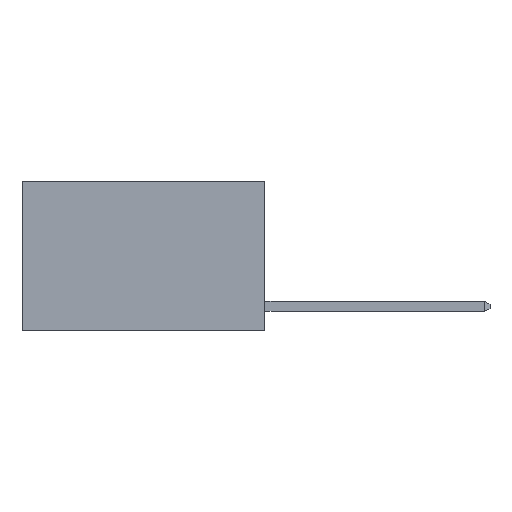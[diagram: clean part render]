
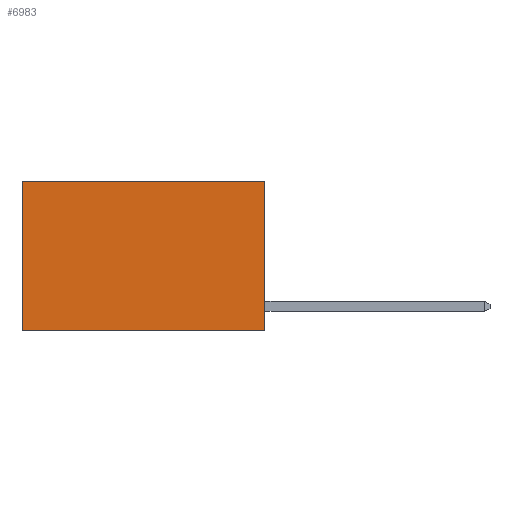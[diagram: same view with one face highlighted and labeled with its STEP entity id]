
A CAD part, left-side view. The second image highlights one B-rep face of the part: STEP entity #6983.
In plain terms, the highlighted planar face has unit normal (-1, 0, 0).
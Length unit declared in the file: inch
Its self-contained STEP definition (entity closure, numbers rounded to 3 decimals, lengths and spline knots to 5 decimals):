
#75 = EDGE_CURVE ( 'NONE', #6960, #1314, #2868, .T. ) ;
#391 = ORIENTED_EDGE ( 'NONE', *, *, #75, .F. ) ;
#564 = EDGE_CURVE ( 'NONE', #5067, #6960, #2175, .T. ) ;
#647 = ORIENTED_EDGE ( 'NONE', *, *, #564, .F. ) ;
#650 = AXIS2_PLACEMENT_3D ( 'NONE', #1604, #6888, #2380 ) ;
#769 = VECTOR ( 'NONE', #7251, 39.37008 ) ;
#1314 = VERTEX_POINT ( 'NONE', #5675 ) ;
#1604 = CARTESIAN_POINT ( 'NONE',  ( 0.2625, 0., 0. ) ) ;
#1895 = EDGE_LOOP ( 'NONE', ( #4285, #391, #647, #6540 ) ) ;
#2159 = EDGE_CURVE ( 'NONE', #8826, #1314, #5031, .T. ) ;
#2175 = LINE ( 'NONE', #5202, #7919 ) ;
#2380 = DIRECTION ( 'NONE',  ( 0., 0., -1. ) ) ;
#2868 = LINE ( 'NONE', #6744, #769 ) ;
#3080 = CARTESIAN_POINT ( 'NONE',  ( 0.2625, 0., -0.37 ) ) ;
#3207 = EDGE_CURVE ( 'NONE', #5067, #8826, #4167, .T. ) ;
#3686 = VECTOR ( 'NONE', #8713, 39.37008 ) ;
#4167 = LINE ( 'NONE', #4323, #3686 ) ;
#4266 = CARTESIAN_POINT ( 'NONE',  ( 0.2625, 0.6, 0. ) ) ;
#4285 = ORIENTED_EDGE ( 'NONE', *, *, #2159, .T. ) ;
#4300 = DIRECTION ( 'NONE',  ( 0., 0., -1. ) ) ;
#4323 = CARTESIAN_POINT ( 'NONE',  ( 0.2625, 0., 0. ) ) ;
#4446 = FACE_OUTER_BOUND ( 'NONE', #1895, .T. ) ;
#5031 = LINE ( 'NONE', #4266, #8787 ) ;
#5067 = VERTEX_POINT ( 'NONE', #8200 ) ;
#5202 = CARTESIAN_POINT ( 'NONE',  ( 0.2625, 0., 0. ) ) ;
#5271 = DIRECTION ( 'NONE',  ( 0., 0., -1. ) ) ;
#5675 = CARTESIAN_POINT ( 'NONE',  ( 0.2625, 0.6, -0.37 ) ) ;
#6501 = CARTESIAN_POINT ( 'NONE',  ( 0.2625, 0.6, 0. ) ) ;
#6540 = ORIENTED_EDGE ( 'NONE', *, *, #3207, .T. ) ;
#6744 = CARTESIAN_POINT ( 'NONE',  ( 0.2625, 0., -0.37 ) ) ;
#6888 = DIRECTION ( 'NONE',  ( 1., 0., 0. ) ) ;
#6960 = VERTEX_POINT ( 'NONE', #3080 ) ;
#6983 = ADVANCED_FACE ( 'NONE', ( #4446 ), #9751, .F. ) ;
#7251 = DIRECTION ( 'NONE',  ( 0., 1., 0. ) ) ;
#7919 = VECTOR ( 'NONE', #5271, 39.37008 ) ;
#8200 = CARTESIAN_POINT ( 'NONE',  ( 0.2625, 0., 0. ) ) ;
#8713 = DIRECTION ( 'NONE',  ( 0., 1., 0. ) ) ;
#8787 = VECTOR ( 'NONE', #4300, 39.37008 ) ;
#8826 = VERTEX_POINT ( 'NONE', #6501 ) ;
#9751 = PLANE ( 'NONE',  #650 ) ;
